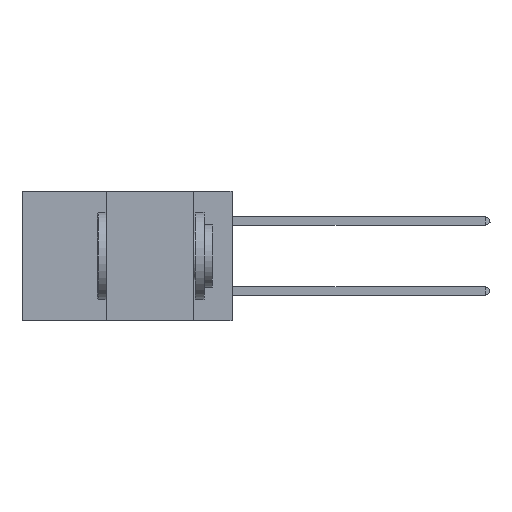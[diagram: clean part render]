
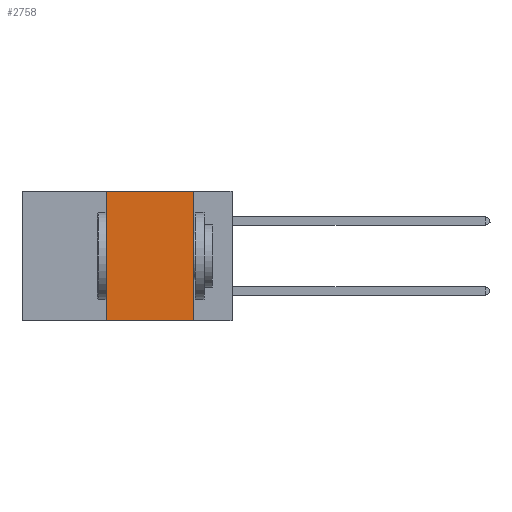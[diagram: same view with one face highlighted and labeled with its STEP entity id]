
A CAD part, left-side view. The second image highlights one B-rep face of the part: STEP entity #2758.
In plain terms, the highlighted planar face has unit normal (-1, 0, 0).
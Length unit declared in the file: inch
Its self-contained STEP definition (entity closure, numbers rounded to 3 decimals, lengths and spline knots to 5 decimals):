
#200 = CARTESIAN_POINT ( 'NONE',  ( 0., 0.11, 0. ) ) ;
#1131 = ORIENTED_EDGE ( 'NONE', *, *, #8596, .F. ) ;
#1266 = ORIENTED_EDGE ( 'NONE', *, *, #13448, .F. ) ;
#1287 = PLANE ( 'NONE',  #11596 ) ;
#1454 = LINE ( 'NONE', #7052, #12578 ) ;
#1517 = ORIENTED_EDGE ( 'NONE', *, *, #6075, .F. ) ;
#1526 = CARTESIAN_POINT ( 'NONE',  ( 0., 0.11, -0.37 ) ) ;
#1530 = ORIENTED_EDGE ( 'NONE', *, *, #9364, .T. ) ;
#2650 = LINE ( 'NONE', #12520, #14710 ) ;
#2758 = ADVANCED_FACE ( 'NONE', ( #13764 ), #1287, .F. ) ;
#3563 = VECTOR ( 'NONE', #4859, 39.37008 ) ;
#3627 = CARTESIAN_POINT ( 'NONE',  ( 0., 0.6, 0. ) ) ;
#4859 = DIRECTION ( 'NONE',  ( 0., -1., 0. ) ) ;
#5695 = VERTEX_POINT ( 'NONE', #14376 ) ;
#6075 = EDGE_CURVE ( 'NONE', #13286, #5695, #1454, .T. ) ;
#6377 = VERTEX_POINT ( 'NONE', #1526 ) ;
#7052 = CARTESIAN_POINT ( 'NONE',  ( 0., 0.36, 0. ) ) ;
#7352 = VECTOR ( 'NONE', #12182, 39.37008 ) ;
#7959 = DIRECTION ( 'NONE',  ( 0., -1., 0. ) ) ;
#8596 = EDGE_CURVE ( 'NONE', #14747, #6377, #10423, .T. ) ;
#8961 = CARTESIAN_POINT ( 'NONE',  ( 0., 0.11, 0. ) ) ;
#9364 = EDGE_CURVE ( 'NONE', #13286, #6377, #2650, .T. ) ;
#9784 = LINE ( 'NONE', #3627, #3563 ) ;
#10423 = LINE ( 'NONE', #200, #7352 ) ;
#11596 = AXIS2_PLACEMENT_3D ( 'NONE', #12409, #12210, #12195 ) ;
#12182 = DIRECTION ( 'NONE',  ( 0., 0., -1. ) ) ;
#12195 = DIRECTION ( 'NONE',  ( 0., 0., -1. ) ) ;
#12210 = DIRECTION ( 'NONE',  ( 1., 0., 0. ) ) ;
#12409 = CARTESIAN_POINT ( 'NONE',  ( 0., 0.6, 0. ) ) ;
#12520 = CARTESIAN_POINT ( 'NONE',  ( 0., 0.6, -0.37 ) ) ;
#12578 = VECTOR ( 'NONE', #15083, 39.37008 ) ;
#12787 = EDGE_LOOP ( 'NONE', ( #1131, #1266, #1517, #1530 ) ) ;
#13286 = VERTEX_POINT ( 'NONE', #13784 ) ;
#13448 = EDGE_CURVE ( 'NONE', #5695, #14747, #9784, .T. ) ;
#13764 = FACE_OUTER_BOUND ( 'NONE', #12787, .T. ) ;
#13784 = CARTESIAN_POINT ( 'NONE',  ( 0., 0.36, -0.37 ) ) ;
#14376 = CARTESIAN_POINT ( 'NONE',  ( 0., 0.36, 0. ) ) ;
#14710 = VECTOR ( 'NONE', #7959, 39.37008 ) ;
#14747 = VERTEX_POINT ( 'NONE', #8961 ) ;
#15083 = DIRECTION ( 'NONE',  ( 0., 0., 1. ) ) ;
